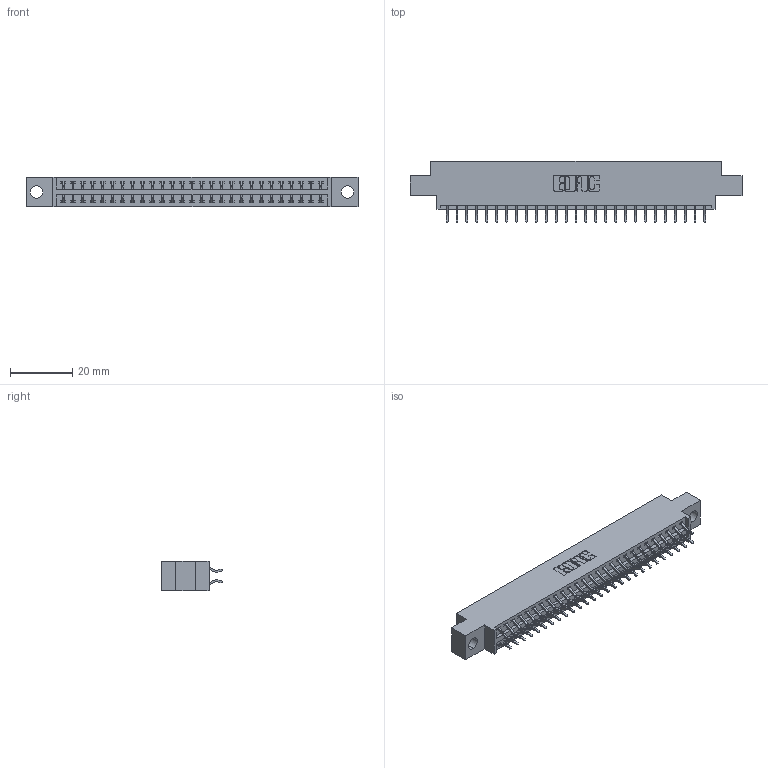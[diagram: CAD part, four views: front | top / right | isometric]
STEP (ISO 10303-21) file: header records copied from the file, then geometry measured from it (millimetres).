
FILE_DESCRIPTION (( 'STEP AP203' ), '1' );
FILE_NAME ('396-054-556-804.STEP', '2018-09-08T08:30:40', ( '' ), ( '' ), 'SwSTEP 2.0', 'SolidWorks 2016', '' );
FILE_SCHEMA (( 'CONFIG_CONTROL_DESIGN' ));
Length unit declared in the file: inch
Products named in the file (3): 396-054-556-804; 346 Part_0.170 Offset - 0.156 Dia-TH; 345-292-001_556 Tail
Assembly tree (55 placements, depth 2):
  396-054-556-804
    346 Part_0.170 Offset - 0.156 Dia-TH
    345-292-001_556 Tail  x54
Bounding box: 106.3 x 19.57 x 9.4 mm (x, y, z)
Volume: 10004.4 mm3; surface area: 13458.7 mm2
Topology: 55 solids, 55 shells, 3258 faces, 9683 edges, 6382 vertices
Faces by surface type: plane 2186, cylinder 1072
Entity records: 19995 total; most frequent: CARTESIAN_POINT 3332, ORIENTED_EDGE 3254, DIRECTION 2975, EDGE_CURVE 1627, VECTOR 1379, LINE 1379, VERTEX_POINT 1082, AXIS2_PLACEMENT_3D 798
